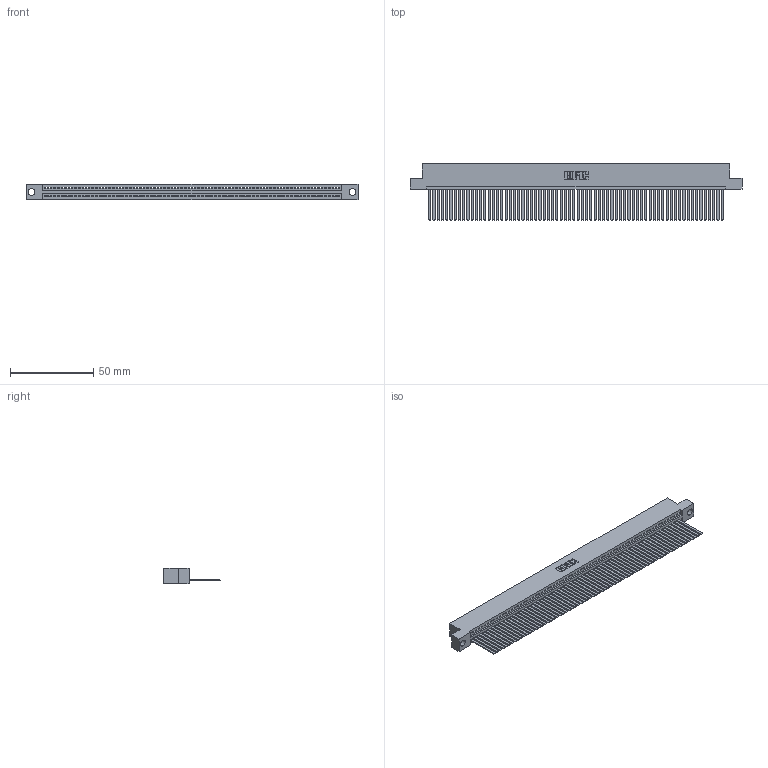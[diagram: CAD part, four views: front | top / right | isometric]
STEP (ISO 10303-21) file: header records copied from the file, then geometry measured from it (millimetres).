
FILE_DESCRIPTION (( 'STEP AP203' ), '1' );
FILE_NAME ('345-070-544-104.STEP', '2019-10-12T18:31:18', ( '' ), ( '' ), 'SwSTEP 2.0', 'SolidWorks 2016', '' );
FILE_SCHEMA (( 'CONFIG_CONTROL_DESIGN' ));
Length unit declared in the file: inch
Products named in the file (3): 345-292-001_345-293-144; 345 Part_Flush Mounting Lugs - 0.156 Dia-TH; 345-070-544-104
Assembly tree (71 placements, depth 2):
  345-070-544-104
    345 Part_Flush Mounting Lugs - 0.156 Dia-TH
    345-292-001_345-293-144  x70
Bounding box: 199.01 x 33.96 x 9.4 mm (x, y, z)
Volume: 19854.3 mm3; surface area: 29007.6 mm2
Topology: 71 solids, 71 shells, 3766 faces, 11401 edges, 7506 vertices
Faces by surface type: plane 2600, cylinder 1166
Entity records: 48733 total; most frequent: ORIENTED_EDGE 8450, CARTESIAN_POINT 8446, DIRECTION 7333, EDGE_CURVE 4225, VECTOR 3817, LINE 3817, VERTEX_POINT 2814, AXIS2_PLACEMENT_3D 1758
